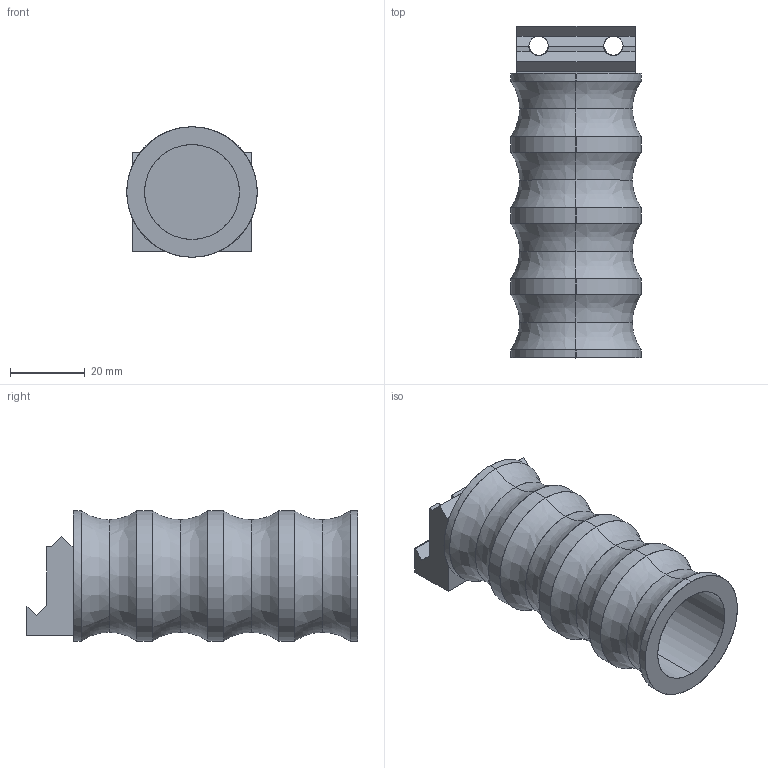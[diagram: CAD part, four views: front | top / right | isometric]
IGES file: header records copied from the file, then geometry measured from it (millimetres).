
Start section: SolidWorks IGES file using analytic representation for surfaces
Global section: file name: ForeGrip.IGS; native system: SolidWorks 2012; preprocessor: SolidWorks 2012; author: BILAL; date: 120422.211344; units: inch
Bounding box: 34.92 x 88.9 x 34.92 mm (x, y, z)
Surface area: 17371.7 mm2 (no closed solid volume)
Topology: 0 solids, 0 shells, 60 faces, 596 edges, 596 vertices
Faces by surface type: bspline 44, revolution 16
